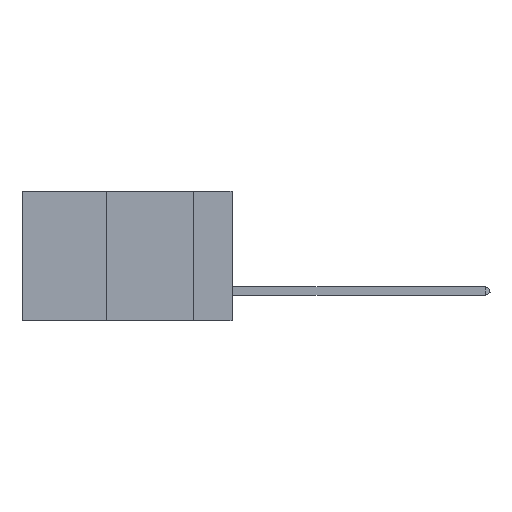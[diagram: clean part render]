
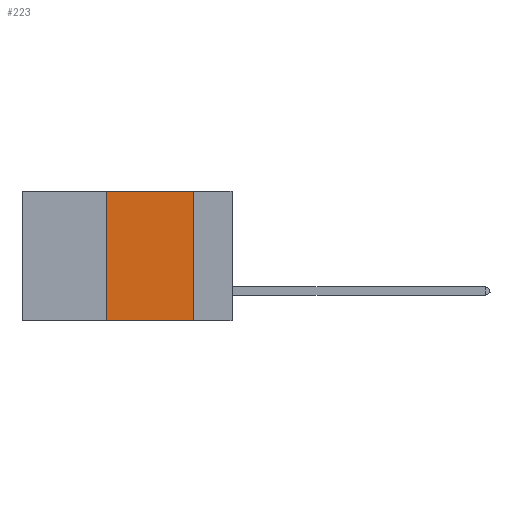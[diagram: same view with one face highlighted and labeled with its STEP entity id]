
A CAD part, left-side view. The second image highlights one B-rep face of the part: STEP entity #223.
In plain terms, the highlighted planar face has unit normal (-1, 0, 0).
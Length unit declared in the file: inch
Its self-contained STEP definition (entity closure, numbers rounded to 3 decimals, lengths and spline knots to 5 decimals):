
#223 = ADVANCED_FACE ( 'NONE', ( #4135 ), #18499, .F. ) ;
#1589 = CARTESIAN_POINT ( 'NONE',  ( 0., 0.36, -0.37 ) ) ;
#2539 = DIRECTION ( 'NONE',  ( 0., 0., -1. ) ) ;
#2737 = ORIENTED_EDGE ( 'NONE', *, *, #8072, .F. ) ;
#3614 = CARTESIAN_POINT ( 'NONE',  ( 0., 0.11, 0. ) ) ;
#3817 = VECTOR ( 'NONE', #17866, 39.37008 ) ;
#4135 = FACE_OUTER_BOUND ( 'NONE', #12039, .T. ) ;
#4206 = VERTEX_POINT ( 'NONE', #1589 ) ;
#4252 = CARTESIAN_POINT ( 'NONE',  ( 0., 0.36, 0. ) ) ;
#4334 = DIRECTION ( 'NONE',  ( 0., 0., 1. ) ) ;
#4942 = LINE ( 'NONE', #4252, #13192 ) ;
#5862 = DIRECTION ( 'NONE',  ( 0., -1., 0. ) ) ;
#7124 = ORIENTED_EDGE ( 'NONE', *, *, #8447, .F. ) ;
#7294 = DIRECTION ( 'NONE',  ( 0., 0., -1. ) ) ;
#7841 = ORIENTED_EDGE ( 'NONE', *, *, #18883, .F. ) ;
#8072 = EDGE_CURVE ( 'NONE', #20583, #22364, #21572, .T. ) ;
#8436 = CARTESIAN_POINT ( 'NONE',  ( 0., 0.36, 0. ) ) ;
#8447 = EDGE_CURVE ( 'NONE', #4206, #20583, #4942, .T. ) ;
#8704 = CARTESIAN_POINT ( 'NONE',  ( 0., 0.6, 0. ) ) ;
#9472 = CARTESIAN_POINT ( 'NONE',  ( 0., 0.6, -0.37 ) ) ;
#12039 = EDGE_LOOP ( 'NONE', ( #7841, #2737, #7124, #15669 ) ) ;
#12215 = VECTOR ( 'NONE', #7294, 39.37008 ) ;
#12754 = LINE ( 'NONE', #16184, #12215 ) ;
#12909 = CARTESIAN_POINT ( 'NONE',  ( 0., 0.11, -0.37 ) ) ;
#13192 = VECTOR ( 'NONE', #4334, 39.37008 ) ;
#14820 = CARTESIAN_POINT ( 'NONE',  ( 0., 0.6, 0. ) ) ;
#15474 = VECTOR ( 'NONE', #5862, 39.37008 ) ;
#15669 = ORIENTED_EDGE ( 'NONE', *, *, #20834, .T. ) ;
#16184 = CARTESIAN_POINT ( 'NONE',  ( 0., 0.11, 0. ) ) ;
#17009 = DIRECTION ( 'NONE',  ( 1., 0., 0. ) ) ;
#17866 = DIRECTION ( 'NONE',  ( 0., -1., 0. ) ) ;
#18499 = PLANE ( 'NONE',  #23056 ) ;
#18883 = EDGE_CURVE ( 'NONE', #22364, #19965, #12754, .T. ) ;
#19965 = VERTEX_POINT ( 'NONE', #12909 ) ;
#20583 = VERTEX_POINT ( 'NONE', #8436 ) ;
#20834 = EDGE_CURVE ( 'NONE', #4206, #19965, #23284, .T. ) ;
#21572 = LINE ( 'NONE', #8704, #3817 ) ;
#22364 = VERTEX_POINT ( 'NONE', #3614 ) ;
#23056 = AXIS2_PLACEMENT_3D ( 'NONE', #14820, #17009, #2539 ) ;
#23284 = LINE ( 'NONE', #9472, #15474 ) ;
